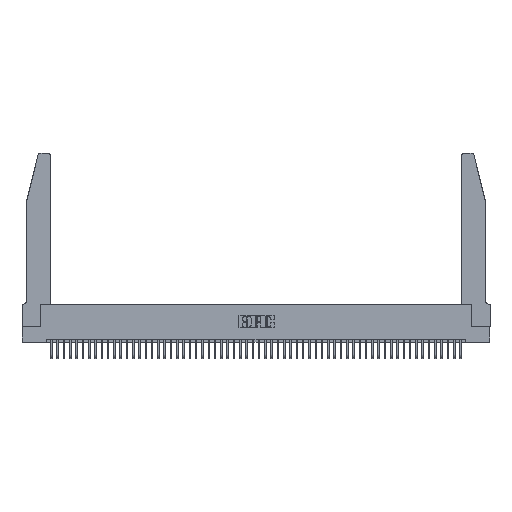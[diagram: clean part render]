
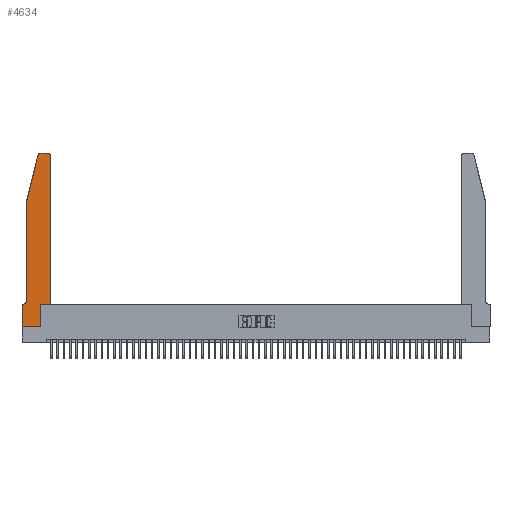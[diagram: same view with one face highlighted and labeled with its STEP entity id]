
A CAD part, top view. The second image highlights one B-rep face of the part: STEP entity #4634.
In plain terms, the highlighted planar face has unit normal (0, 0, 1).
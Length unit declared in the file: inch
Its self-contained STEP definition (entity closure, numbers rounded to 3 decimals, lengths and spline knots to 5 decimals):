
#120 = LINE ( 'NONE', #19018, #9559 ) ;
#1960 = CARTESIAN_POINT ( 'NONE',  ( 0.4205, 2.75, 0.37 ) ) ;
#2955 = EDGE_CURVE ( 'NONE', #34326, #41063, #35841, .T. ) ;
#3615 = CARTESIAN_POINT ( 'NONE',  ( 0.4505, 2.72, 0.37 ) ) ;
#3628 = LINE ( 'NONE', #34803, #13007 ) ;
#3993 = EDGE_CURVE ( 'NONE', #44158, #50109, #37545, .T. ) ;
#4020 = ORIENTED_EDGE ( 'NONE', *, *, #29383, .T. ) ;
#4634 = ADVANCED_FACE ( 'NONE', ( #48619 ), #18320, .T. ) ;
#6123 = EDGE_CURVE ( 'NONE', #51043, #15617, #120, .T. ) ;
#7009 = LINE ( 'NONE', #9142, #47803 ) ;
#7326 = AXIS2_PLACEMENT_3D ( 'NONE', #23178, #50617, #27102 ) ;
#7609 = CARTESIAN_POINT ( 'NONE',  ( 0.0755, 0.42, 0.37 ) ) ;
#9142 = CARTESIAN_POINT ( 'NONE',  ( 0.4505, 0.35, 0.37 ) ) ;
#9559 = VECTOR ( 'NONE', #46510, 39.37008 ) ;
#11793 = VECTOR ( 'NONE', #46884, 39.37008 ) ;
#11854 = DIRECTION ( 'NONE',  ( 0., 0., 1. ) ) ;
#12376 = EDGE_LOOP ( 'NONE', ( #33659, #29841, #29323, #31082, #20145, #13604, #15185, #49418, #15531, #41208, #4020, #45128 ) ) ;
#12418 = EDGE_CURVE ( 'NONE', #25173, #51043, #28660, .T. ) ;
#13007 = VECTOR ( 'NONE', #42746, 39.37008 ) ;
#13289 = LINE ( 'NONE', #41676, #33037 ) ;
#13604 = ORIENTED_EDGE ( 'NONE', *, *, #18849, .T. ) ;
#13777 = CARTESIAN_POINT ( 'NONE',  ( 0.284, 2.75, 0.37 ) ) ;
#14012 = AXIS2_PLACEMENT_3D ( 'NONE', #14338, #41913, #18379 ) ;
#14094 = DIRECTION ( 'NONE',  ( 0., 1., 0. ) ) ;
#14338 = CARTESIAN_POINT ( 'NONE',  ( 0.4205, 2.72, 0.37 ) ) ;
#14610 = LINE ( 'NONE', #42430, #35571 ) ;
#15002 = CARTESIAN_POINT ( 'NONE',  ( 0.0755, 0.35, 0.37 ) ) ;
#15185 = ORIENTED_EDGE ( 'NONE', *, *, #12418, .T. ) ;
#15352 = VECTOR ( 'NONE', #46538, 39.37008 ) ;
#15531 = ORIENTED_EDGE ( 'NONE', *, *, #20431, .T. ) ;
#15617 = VERTEX_POINT ( 'NONE', #27549 ) ;
#17132 = VERTEX_POINT ( 'NONE', #40140 ) ;
#18320 = PLANE ( 'NONE',  #27983 ) ;
#18379 = DIRECTION ( 'NONE',  ( 1., 0., 0. ) ) ;
#18832 = CARTESIAN_POINT ( 'NONE',  ( 0.4505, 0.35, 0.37 ) ) ;
#18849 = EDGE_CURVE ( 'NONE', #17132, #25173, #46783, .T. ) ;
#18898 = DIRECTION ( 'NONE',  ( 1., 0., 0. ) ) ;
#19018 = CARTESIAN_POINT ( 'NONE',  ( 0., 0., 0.37 ) ) ;
#19080 = CIRCLE ( 'NONE', #7326, 0.07 ) ;
#19491 = CARTESIAN_POINT ( 'NONE',  ( 0.2865, 0.35, 0.37 ) ) ;
#20145 = ORIENTED_EDGE ( 'NONE', *, *, #34594, .T. ) ;
#20431 = EDGE_CURVE ( 'NONE', #15617, #26082, #13289, .T. ) ;
#20557 = LINE ( 'NONE', #35874, #40200 ) ;
#21324 = DIRECTION ( 'NONE',  ( 0., -1., 0. ) ) ;
#22290 = DIRECTION ( 'NONE',  ( 0., 0., 1. ) ) ;
#22334 = AXIS2_PLACEMENT_3D ( 'NONE', #35448, #11854, #39410 ) ;
#23178 = CARTESIAN_POINT ( 'NONE',  ( 0.0055, 0.42, 0.37 ) ) ;
#23769 = VERTEX_POINT ( 'NONE', #18832 ) ;
#25173 = VERTEX_POINT ( 'NONE', #51184 ) ;
#26082 = VERTEX_POINT ( 'NONE', #19491 ) ;
#27102 = DIRECTION ( 'NONE',  ( -1., 0., 0. ) ) ;
#27549 = CARTESIAN_POINT ( 'NONE',  ( 0.2865, 0., 0.37 ) ) ;
#27983 = AXIS2_PLACEMENT_3D ( 'NONE', #41689, #22290, #49763 ) ;
#28364 = EDGE_CURVE ( 'NONE', #26082, #23769, #14610, .T. ) ;
#28660 = LINE ( 'NONE', #40882, #37812 ) ;
#29323 = ORIENTED_EDGE ( 'NONE', *, *, #37515, .T. ) ;
#29383 = EDGE_CURVE ( 'NONE', #23769, #44158, #7009, .T. ) ;
#29841 = ORIENTED_EDGE ( 'NONE', *, *, #2955, .T. ) ;
#30994 = VERTEX_POINT ( 'NONE', #32473 ) ;
#31082 = ORIENTED_EDGE ( 'NONE', *, *, #37527, .T. ) ;
#32473 = CARTESIAN_POINT ( 'NONE',  ( 0.0755, 2., 0.37 ) ) ;
#33037 = VECTOR ( 'NONE', #14094, 39.37008 ) ;
#33659 = ORIENTED_EDGE ( 'NONE', *, *, #46715, .T. ) ;
#34326 = VERTEX_POINT ( 'NONE', #13777 ) ;
#34594 = EDGE_CURVE ( 'NONE', #44792, #17132, #19080, .T. ) ;
#34803 = CARTESIAN_POINT ( 'NONE',  ( 0.0755, 2., 0.37 ) ) ;
#35448 = CARTESIAN_POINT ( 'NONE',  ( 0.284, 2.72, 0.37 ) ) ;
#35571 = VECTOR ( 'NONE', #18898, 39.37008 ) ;
#35841 = CIRCLE ( 'NONE', #22334, 0.03 ) ;
#35874 = CARTESIAN_POINT ( 'NONE',  ( 0.2605, 2.75, 0.37 ) ) ;
#36898 = DIRECTION ( 'NONE',  ( 0., 1., 0. ) ) ;
#37515 = EDGE_CURVE ( 'NONE', #41063, #30994, #3628, .T. ) ;
#37527 = EDGE_CURVE ( 'NONE', #30994, #44792, #43261, .T. ) ;
#37545 = CIRCLE ( 'NONE', #14012, 0.03 ) ;
#37812 = VECTOR ( 'NONE', #21324, 39.37008 ) ;
#39410 = DIRECTION ( 'NONE',  ( 1., 0., 0. ) ) ;
#39849 = DIRECTION ( 'NONE',  ( -1., 0., 0. ) ) ;
#40140 = CARTESIAN_POINT ( 'NONE',  ( 0.0055, 0.35, 0.37 ) ) ;
#40200 = VECTOR ( 'NONE', #39849, 39.37008 ) ;
#40882 = CARTESIAN_POINT ( 'NONE',  ( 0., 0., 0.37 ) ) ;
#41063 = VERTEX_POINT ( 'NONE', #48098 ) ;
#41208 = ORIENTED_EDGE ( 'NONE', *, *, #28364, .T. ) ;
#41676 = CARTESIAN_POINT ( 'NONE',  ( 0.2865, 0.35, 0.37 ) ) ;
#41689 = CARTESIAN_POINT ( 'NONE',  ( 0., 0.35, 0.37 ) ) ;
#41913 = DIRECTION ( 'NONE',  ( 0., 0., 1. ) ) ;
#42430 = CARTESIAN_POINT ( 'NONE',  ( 0.4505, 0.35, 0.37 ) ) ;
#42746 = DIRECTION ( 'NONE',  ( -0.239, -0.971, 0. ) ) ;
#42928 = CARTESIAN_POINT ( 'NONE',  ( 0.0755, 2., 0.37 ) ) ;
#43261 = LINE ( 'NONE', #42928, #11793 ) ;
#44158 = VERTEX_POINT ( 'NONE', #3615 ) ;
#44792 = VERTEX_POINT ( 'NONE', #7609 ) ;
#45128 = ORIENTED_EDGE ( 'NONE', *, *, #3993, .T. ) ;
#46510 = DIRECTION ( 'NONE',  ( 1., 0., 0. ) ) ;
#46538 = DIRECTION ( 'NONE',  ( -1., 0., 0. ) ) ;
#46715 = EDGE_CURVE ( 'NONE', #50109, #34326, #20557, .T. ) ;
#46783 = LINE ( 'NONE', #15002, #15352 ) ;
#46884 = DIRECTION ( 'NONE',  ( 0., -1., 0. ) ) ;
#47045 = CARTESIAN_POINT ( 'NONE',  ( 0., 0., 0.37 ) ) ;
#47803 = VECTOR ( 'NONE', #36898, 39.37008 ) ;
#48098 = CARTESIAN_POINT ( 'NONE',  ( 0.25487, 2.72718, 0.37 ) ) ;
#48619 = FACE_OUTER_BOUND ( 'NONE', #12376, .T. ) ;
#49418 = ORIENTED_EDGE ( 'NONE', *, *, #6123, .T. ) ;
#49763 = DIRECTION ( 'NONE',  ( 1., 0., 0. ) ) ;
#50109 = VERTEX_POINT ( 'NONE', #1960 ) ;
#50617 = DIRECTION ( 'NONE',  ( 0., 0., -1. ) ) ;
#51043 = VERTEX_POINT ( 'NONE', #47045 ) ;
#51184 = CARTESIAN_POINT ( 'NONE',  ( 0., 0.35, 0.37 ) ) ;
